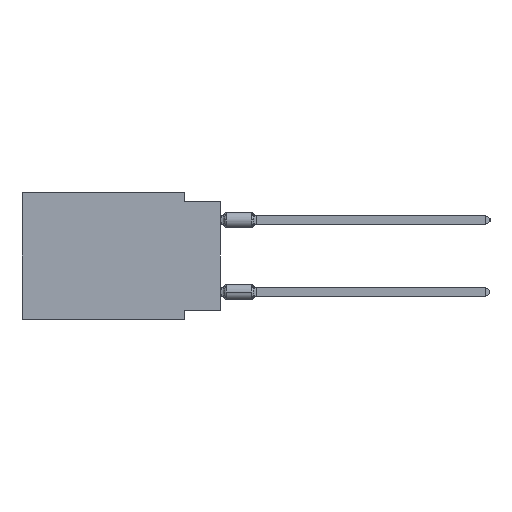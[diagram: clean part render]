
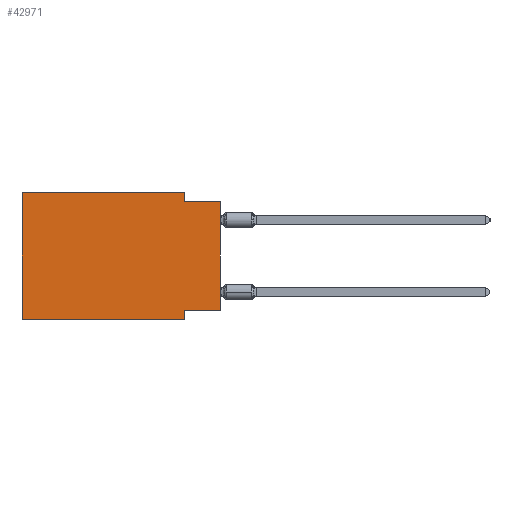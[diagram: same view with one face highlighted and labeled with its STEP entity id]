
A CAD part, left-side view. The second image highlights one B-rep face of the part: STEP entity #42971.
In plain terms, the highlighted planar face has unit normal (-1, 0, 0).
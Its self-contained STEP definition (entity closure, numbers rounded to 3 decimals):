
#349 = EDGE_LOOP ( 'NONE', ( #18444, #46783, #26589, #27638, #5736, #2234, #9976, #39671 ) ) ;
#656 = DIRECTION ( 'NONE',  ( 0., 0., -1. ) ) ;
#1009 = DIRECTION ( 'NONE',  ( 0., -1., 0. ) ) ;
#2061 = VECTOR ( 'NONE', #16324, 1000. ) ;
#2234 = ORIENTED_EDGE ( 'NONE', *, *, #66391, .T. ) ;
#2363 = EDGE_CURVE ( 'NONE', #25757, #36215, #34524, .T. ) ;
#4793 = VERTEX_POINT ( 'NONE', #30859 ) ;
#5195 = CARTESIAN_POINT ( 'NONE',  ( 0., 0., -0.635 ) ) ;
#5736 = ORIENTED_EDGE ( 'NONE', *, *, #54965, .F. ) ;
#9585 = CARTESIAN_POINT ( 'NONE',  ( 0., 13.97, 0. ) ) ;
#9900 = CARTESIAN_POINT ( 'NONE',  ( 0., 0., -8.255 ) ) ;
#9976 = ORIENTED_EDGE ( 'NONE', *, *, #39685, .F. ) ;
#10067 = VECTOR ( 'NONE', #50669, 1000. ) ;
#10388 = VECTOR ( 'NONE', #29162, 1000. ) ;
#11130 = VECTOR ( 'NONE', #54756, 1000. ) ;
#11311 = EDGE_CURVE ( 'NONE', #36215, #18567, #27308, .T. ) ;
#11762 = DIRECTION ( 'NONE',  ( 0., 0., 1. ) ) ;
#12178 = LINE ( 'NONE', #34637, #10067 ) ;
#16324 = DIRECTION ( 'NONE',  ( 0., 0., 1. ) ) ;
#16962 = CARTESIAN_POINT ( 'NONE',  ( 0., 0., -0.635 ) ) ;
#18444 = ORIENTED_EDGE ( 'NONE', *, *, #54680, .T. ) ;
#18567 = VERTEX_POINT ( 'NONE', #5195 ) ;
#19331 = EDGE_CURVE ( 'NONE', #47845, #25757, #23100, .T. ) ;
#22728 = CARTESIAN_POINT ( 'NONE',  ( 0., 13.97, 0. ) ) ;
#22812 = LINE ( 'NONE', #38852, #32723 ) ;
#23096 = PLANE ( 'NONE',  #63625 ) ;
#23100 = LINE ( 'NONE', #49129, #28971 ) ;
#24522 = CARTESIAN_POINT ( 'NONE',  ( 0., 2.54, 0. ) ) ;
#25757 = VERTEX_POINT ( 'NONE', #54442 ) ;
#26346 = LINE ( 'NONE', #48091, #35049 ) ;
#26530 = CARTESIAN_POINT ( 'NONE',  ( 0., 2.54, -0.635 ) ) ;
#26589 = ORIENTED_EDGE ( 'NONE', *, *, #2363, .F. ) ;
#27048 = VERTEX_POINT ( 'NONE', #33150 ) ;
#27308 = LINE ( 'NONE', #16962, #11130 ) ;
#27638 = ORIENTED_EDGE ( 'NONE', *, *, #19331, .F. ) ;
#28971 = VECTOR ( 'NONE', #1009, 1000. ) ;
#29162 = DIRECTION ( 'NONE',  ( 0., 0., -1. ) ) ;
#30662 = EDGE_CURVE ( 'NONE', #4793, #58532, #36647, .T. ) ;
#30859 = CARTESIAN_POINT ( 'NONE',  ( 0., 0., -8.255 ) ) ;
#32723 = VECTOR ( 'NONE', #11762, 1000. ) ;
#33078 = FACE_OUTER_BOUND ( 'NONE', #349, .T. ) ;
#33150 = CARTESIAN_POINT ( 'NONE',  ( 0., 13.97, -8.89 ) ) ;
#34524 = LINE ( 'NONE', #24522, #10388 ) ;
#34637 = CARTESIAN_POINT ( 'NONE',  ( 0., 2.54, -8.89 ) ) ;
#35049 = VECTOR ( 'NONE', #65202, 1000. ) ;
#36215 = VERTEX_POINT ( 'NONE', #26530 ) ;
#36647 = LINE ( 'NONE', #9900, #58346 ) ;
#38065 = LINE ( 'NONE', #9585, #2061 ) ;
#38240 = CARTESIAN_POINT ( 'NONE',  ( 0., 2.54, -8.255 ) ) ;
#38852 = CARTESIAN_POINT ( 'NONE',  ( 0., 0., 0. ) ) ;
#39671 = ORIENTED_EDGE ( 'NONE', *, *, #30662, .F. ) ;
#39685 = EDGE_CURVE ( 'NONE', #58532, #48891, #12178, .T. ) ;
#41527 = CARTESIAN_POINT ( 'NONE',  ( 0., 2.54, -8.89 ) ) ;
#42971 = ADVANCED_FACE ( 'NONE', ( #33078 ), #23096, .F. ) ;
#44310 = CARTESIAN_POINT ( 'NONE',  ( 0., 13.97, 0. ) ) ;
#46783 = ORIENTED_EDGE ( 'NONE', *, *, #11311, .F. ) ;
#47845 = VERTEX_POINT ( 'NONE', #44310 ) ;
#48091 = CARTESIAN_POINT ( 'NONE',  ( 0., 13.97, -8.89 ) ) ;
#48891 = VERTEX_POINT ( 'NONE', #41527 ) ;
#49129 = CARTESIAN_POINT ( 'NONE',  ( 0., 13.97, 0. ) ) ;
#50669 = DIRECTION ( 'NONE',  ( 0., 0., -1. ) ) ;
#54442 = CARTESIAN_POINT ( 'NONE',  ( 0., 2.54, 0. ) ) ;
#54680 = EDGE_CURVE ( 'NONE', #4793, #18567, #22812, .T. ) ;
#54756 = DIRECTION ( 'NONE',  ( 0., -1., 0. ) ) ;
#54965 = EDGE_CURVE ( 'NONE', #27048, #47845, #38065, .T. ) ;
#58346 = VECTOR ( 'NONE', #58404, 1000. ) ;
#58404 = DIRECTION ( 'NONE',  ( 0., 1., 0. ) ) ;
#58532 = VERTEX_POINT ( 'NONE', #38240 ) ;
#60532 = DIRECTION ( 'NONE',  ( 1., 0., 0. ) ) ;
#63625 = AXIS2_PLACEMENT_3D ( 'NONE', #22728, #60532, #656 ) ;
#65202 = DIRECTION ( 'NONE',  ( 0., -1., 0. ) ) ;
#66391 = EDGE_CURVE ( 'NONE', #27048, #48891, #26346, .T. ) ;
